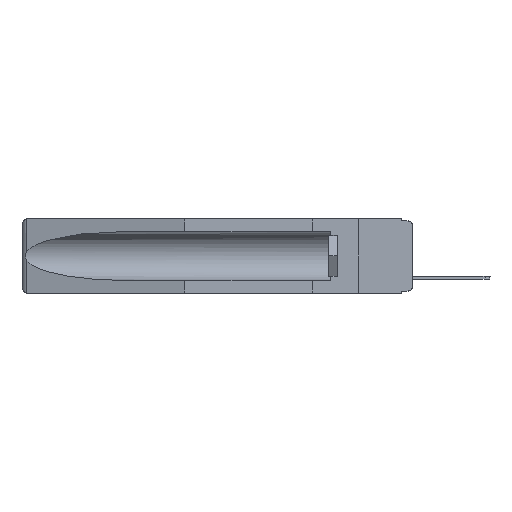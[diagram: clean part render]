
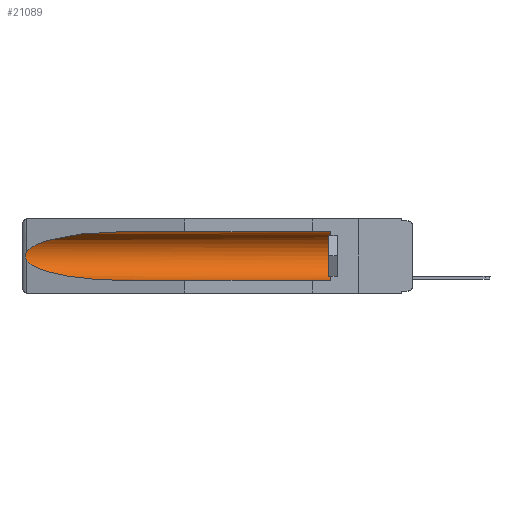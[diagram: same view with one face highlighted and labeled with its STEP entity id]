
A CAD part, left-side view. The second image highlights one B-rep face of the part: STEP entity #21089.
In plain terms, the highlighted cylindrical face has radius 2.857 mm (diameter 5.715 mm), a partial arc.
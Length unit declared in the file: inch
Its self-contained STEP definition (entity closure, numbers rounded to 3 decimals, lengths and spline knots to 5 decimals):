
#583 = DIRECTION ( 'NONE',  ( 0., 0., 1. ) ) ;
#661 = CARTESIAN_POINT ( 'NONE',  ( 0.155, -0.30754, -0.1715 ) ) ;
#1788 = CARTESIAN_POINT ( 'NONE',  ( 0.25451, 1.48313, -0.24835 ) ) ;
#1885 = CARTESIAN_POINT ( 'NONE',  ( 0.2673, 1.5327, -0.16383 ) ) ;
#2189 = CARTESIAN_POINT ( 'NONE',  ( 0.26537, 1.52718, -0.14972 ) ) ;
#2325 = ORIENTED_EDGE ( 'NONE', *, *, #4115, .T. ) ;
#2383 = VERTEX_POINT ( 'NONE', #22109 ) ;
#2957 = DIRECTION ( 'NONE',  ( 0., 1., 0. ) ) ;
#3139 = DIRECTION ( 'NONE',  ( 0., -1., 0. ) ) ;
#3516 = DIRECTION ( 'NONE',  ( 0., 1., 0. ) ) ;
#3713 = CARTESIAN_POINT ( 'NONE',  ( 0.2675, 1.53308, -0.17534 ) ) ;
#3966 = ORIENTED_EDGE ( 'NONE', *, *, #12644, .F. ) ;
#4115 = EDGE_CURVE ( 'NONE', #18160, #11167, #16495, .T. ) ;
#4634 = CYLINDRICAL_SURFACE ( 'NONE', #10322, 0.1125 ) ;
#5198 = CARTESIAN_POINT ( 'NONE',  ( 0.155, 1.07973, -0.059 ) ) ;
#5523 = LINE ( 'NONE', #20862, #18567 ) ;
#5731 = LINE ( 'NONE', #6909, #11246 ) ;
#6038 = VERTEX_POINT ( 'NONE', #2189 ) ;
#6758 = DIRECTION ( 'NONE',  ( 0., 0., 1. ) ) ;
#6909 = CARTESIAN_POINT ( 'NONE',  ( 0.155, -0.30754, -0.284 ) ) ;
#8108 = VERTEX_POINT ( 'NONE', #22336 ) ;
#8535 = CARTESIAN_POINT ( 'NONE',  ( 0.26537, 1.52718, -0.14972 ) ) ;
#8874 = EDGE_CURVE ( 'NONE', #11167, #19790, #5523, .T. ) ;
#9810 = DIRECTION ( 'NONE',  ( 0., 1., 0. ) ) ;
#10107 = EDGE_CURVE ( 'NONE', #19790, #6038, #10461, .T. ) ;
#10170 = CARTESIAN_POINT ( 'NONE',  ( 0.155, 0.126, -0.1715 ) ) ;
#10322 = AXIS2_PLACEMENT_3D ( 'NONE', #661, #9810, #583 ) ;
#10461 =( BOUNDED_CURVE ( )  B_SPLINE_CURVE ( 3, ( #5198, #19156, #17603, #8535 ),
 .UNSPECIFIED., .F., .F. ) 
 B_SPLINE_CURVE_WITH_KNOTS ( ( 4, 4 ),
 ( 4.71239, 6.08839 ),
 .UNSPECIFIED. ) 
 CURVE ( )  GEOMETRIC_REPRESENTATION_ITEM ( )  RATIONAL_B_SPLINE_CURVE ( ( 1., 0.848, 0.848, 1. ) ) 
 REPRESENTATION_ITEM ( '' )  );
#10805 = CARTESIAN_POINT ( 'NONE',  ( 0.26597, 1.5296, -0.19026 ) ) ;
#11167 = VERTEX_POINT ( 'NONE', #18389 ) ;
#11246 = VECTOR ( 'NONE', #3516, 39.37008 ) ;
#12506 = CARTESIAN_POINT ( 'NONE',  ( 0.155, 1.07973, -0.284 ) ) ;
#12644 = EDGE_CURVE ( 'NONE', #18160, #2383, #5731, .T. ) ;
#12743 = CARTESIAN_POINT ( 'NONE',  ( 0.2675, 1.53308, -0.16763 ) ) ;
#13658 = EDGE_LOOP ( 'NONE', ( #17851, #20937, #19556, #3966, #2325, #18994 ) ) ;
#14129 = CARTESIAN_POINT ( 'NONE',  ( 0.155, 1.07973, -0.059 ) ) ;
#15454 = B_SPLINE_CURVE_WITH_KNOTS ( 'NONE', 3,
 ( #19806, #17970, #16108, #1885, #12743, #3713, #17890, #21531, #10805, #21686 ),
 .UNSPECIFIED., .F., .F.,
 ( 4, 2, 2, 2, 4 ),
 ( 0., 0.00029, 0.00058, 0.00087, 0.00117 ),
 .UNSPECIFIED. ) ;
#15873 = EDGE_CURVE ( 'NONE', #8108, #2383, #18152, .T. ) ;
#16108 = CARTESIAN_POINT ( 'NONE',  ( 0.26654, 1.53092, -0.15636 ) ) ;
#16495 = CIRCLE ( 'NONE', #21266, 0.1125 ) ;
#17223 = EDGE_CURVE ( 'NONE', #6038, #8108, #15454, .T. ) ;
#17603 = CARTESIAN_POINT ( 'NONE',  ( 0.25451, 1.48313, -0.09465 ) ) ;
#17642 = CARTESIAN_POINT ( 'NONE',  ( 0.21114, 1.30732, -0.284 ) ) ;
#17851 = ORIENTED_EDGE ( 'NONE', *, *, #10107, .T. ) ;
#17890 = CARTESIAN_POINT ( 'NONE',  ( 0.2673, 1.53269, -0.17917 ) ) ;
#17959 = FACE_OUTER_BOUND ( 'NONE', #13658, .T. ) ;
#17970 = CARTESIAN_POINT ( 'NONE',  ( 0.26597, 1.52961, -0.15275 ) ) ;
#18152 =( BOUNDED_CURVE ( )  B_SPLINE_CURVE ( 3, ( #19347, #1788, #17642, #12506 ),
 .UNSPECIFIED., .F., .F. ) 
 B_SPLINE_CURVE_WITH_KNOTS ( ( 4, 4 ),
 ( 0.1948, 1.5708 ),
 .UNSPECIFIED. ) 
 CURVE ( )  GEOMETRIC_REPRESENTATION_ITEM ( )  RATIONAL_B_SPLINE_CURVE ( ( 1., 0.848, 0.848, 1. ) ) 
 REPRESENTATION_ITEM ( '' )  );
#18160 = VERTEX_POINT ( 'NONE', #19997 ) ;
#18389 = CARTESIAN_POINT ( 'NONE',  ( 0.155, 0.126, -0.059 ) ) ;
#18567 = VECTOR ( 'NONE', #2957, 39.37008 ) ;
#18994 = ORIENTED_EDGE ( 'NONE', *, *, #8874, .T. ) ;
#19156 = CARTESIAN_POINT ( 'NONE',  ( 0.21114, 1.30732, -0.059 ) ) ;
#19347 = CARTESIAN_POINT ( 'NONE',  ( 0.26537, 1.52718, -0.19328 ) ) ;
#19556 = ORIENTED_EDGE ( 'NONE', *, *, #15873, .T. ) ;
#19790 = VERTEX_POINT ( 'NONE', #14129 ) ;
#19806 = CARTESIAN_POINT ( 'NONE',  ( 0.26537, 1.52718, -0.14972 ) ) ;
#19997 = CARTESIAN_POINT ( 'NONE',  ( 0.155, 0.126, -0.284 ) ) ;
#20862 = CARTESIAN_POINT ( 'NONE',  ( 0.155, -0.30754, -0.059 ) ) ;
#20937 = ORIENTED_EDGE ( 'NONE', *, *, #17223, .T. ) ;
#21089 = ADVANCED_FACE ( 'NONE', ( #17959 ), #4634, .F. ) ;
#21266 = AXIS2_PLACEMENT_3D ( 'NONE', #10170, #3139, #6758 ) ;
#21531 = CARTESIAN_POINT ( 'NONE',  ( 0.26655, 1.53094, -0.18657 ) ) ;
#21686 = CARTESIAN_POINT ( 'NONE',  ( 0.26537, 1.52718, -0.19328 ) ) ;
#22109 = CARTESIAN_POINT ( 'NONE',  ( 0.155, 1.07973, -0.284 ) ) ;
#22336 = CARTESIAN_POINT ( 'NONE',  ( 0.26537, 1.52718, -0.19328 ) ) ;
